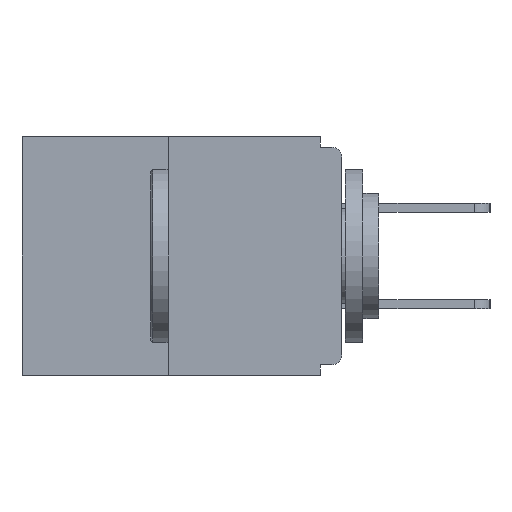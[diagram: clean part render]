
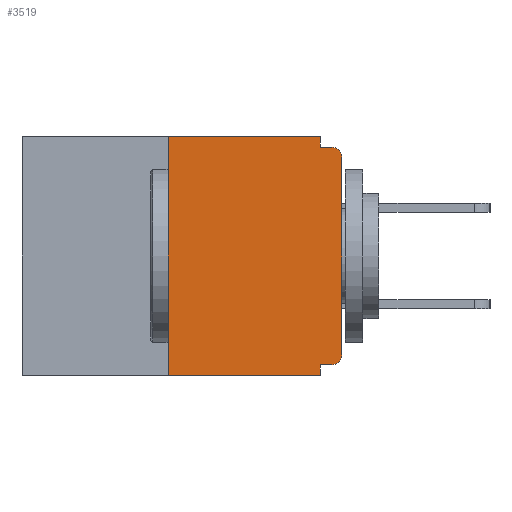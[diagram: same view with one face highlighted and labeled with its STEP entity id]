
A CAD part, left-side view. The second image highlights one B-rep face of the part: STEP entity #3519.
In plain terms, the highlighted planar face has unit normal (-1, 0, 0).
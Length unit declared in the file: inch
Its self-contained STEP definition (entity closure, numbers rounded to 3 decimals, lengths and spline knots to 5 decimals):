
#75 = PLANE ( 'NONE',  #11798 ) ;
#1133 = EDGE_CURVE ( 'NONE', #11866, #6077, #1336, .T. ) ;
#1336 = LINE ( 'NONE', #8271, #6905 ) ;
#1445 = CIRCLE ( 'NONE', #12105, 0.015 ) ;
#1450 = EDGE_CURVE ( 'NONE', #10068, #6450, #13166, .T. ) ;
#1694 = DIRECTION ( 'NONE',  ( 0., 1., 0. ) ) ;
#1868 = AXIS2_PLACEMENT_3D ( 'NONE', #6262, #10805, #14112 ) ;
#1869 = DIRECTION ( 'NONE',  ( -1., 0., 0. ) ) ;
#2560 = CARTESIAN_POINT ( 'NONE',  ( 0., 0., -0.313 ) ) ;
#2639 = ORIENTED_EDGE ( 'NONE', *, *, #13439, .T. ) ;
#2716 = VECTOR ( 'NONE', #14176, 39.37008 ) ;
#2807 = EDGE_LOOP ( 'NONE', ( #3450, #4086, #14605, #4460, #13716, #2639, #9284, #4116, #13426, #13278 ) ) ;
#2814 = CARTESIAN_POINT ( 'NONE',  ( 0., 0.031, 0. ) ) ;
#3253 = VECTOR ( 'NONE', #10194, 39.37008 ) ;
#3293 = LINE ( 'NONE', #13962, #11743 ) ;
#3375 = CARTESIAN_POINT ( 'NONE',  ( 0., 0.25, -0.343 ) ) ;
#3436 = VERTEX_POINT ( 'NONE', #9555 ) ;
#3450 = ORIENTED_EDGE ( 'NONE', *, *, #1450, .F. ) ;
#3519 = ADVANCED_FACE ( 'NONE', ( #8879 ), #75, .F. ) ;
#3564 = DIRECTION ( 'NONE',  ( 0., 0., 1. ) ) ;
#3602 = VERTEX_POINT ( 'NONE', #3375 ) ;
#3792 = CARTESIAN_POINT ( 'NONE',  ( 0., 0.031, -0.343 ) ) ;
#3948 = CARTESIAN_POINT ( 'NONE',  ( 0., 0., -0.015 ) ) ;
#4086 = ORIENTED_EDGE ( 'NONE', *, *, #5072, .F. ) ;
#4116 = ORIENTED_EDGE ( 'NONE', *, *, #10416, .T. ) ;
#4256 = EDGE_CURVE ( 'NONE', #3436, #7676, #9590, .T. ) ;
#4460 = ORIENTED_EDGE ( 'NONE', *, *, #14014, .F. ) ;
#5072 = EDGE_CURVE ( 'NONE', #3602, #10068, #10771, .T. ) ;
#5111 = DIRECTION ( 'NONE',  ( 0., 0., -1. ) ) ;
#5269 = DIRECTION ( 'NONE',  ( 0., 0., -1. ) ) ;
#5365 = VECTOR ( 'NONE', #1694, 39.37008 ) ;
#5390 = VERTEX_POINT ( 'NONE', #5520 ) ;
#5520 = CARTESIAN_POINT ( 'NONE',  ( 0., 0.031, -0.328 ) ) ;
#5783 = DIRECTION ( 'NONE',  ( 1., 0., 0. ) ) ;
#6077 = VERTEX_POINT ( 'NONE', #9287 ) ;
#6115 = EDGE_CURVE ( 'NONE', #11782, #5390, #8964, .T. ) ;
#6226 = DIRECTION ( 'NONE',  ( 0., -1., 0. ) ) ;
#6262 = CARTESIAN_POINT ( 'NONE',  ( 0., 0.015, -0.313 ) ) ;
#6299 = CARTESIAN_POINT ( 'NONE',  ( 0., 0., -0.328 ) ) ;
#6450 = VERTEX_POINT ( 'NONE', #11393 ) ;
#6757 = CARTESIAN_POINT ( 'NONE',  ( 0., 0.46, 0. ) ) ;
#6905 = VECTOR ( 'NONE', #3564, 39.37008 ) ;
#6988 = CARTESIAN_POINT ( 'NONE',  ( 0., 0.46, -0.343 ) ) ;
#7676 = VERTEX_POINT ( 'NONE', #14600 ) ;
#7972 = VECTOR ( 'NONE', #6226, 39.37008 ) ;
#8271 = CARTESIAN_POINT ( 'NONE',  ( 0., 0., 0. ) ) ;
#8824 = CARTESIAN_POINT ( 'NONE',  ( 0., 0.46, 0. ) ) ;
#8879 = FACE_OUTER_BOUND ( 'NONE', #2807, .T. ) ;
#8964 = LINE ( 'NONE', #6299, #5365 ) ;
#9036 = CARTESIAN_POINT ( 'NONE',  ( 0., 0.015, -0.328 ) ) ;
#9061 = EDGE_CURVE ( 'NONE', #3602, #11951, #14658, .T. ) ;
#9284 = ORIENTED_EDGE ( 'NONE', *, *, #1133, .T. ) ;
#9287 = CARTESIAN_POINT ( 'NONE',  ( 0., 0., -0.03 ) ) ;
#9555 = CARTESIAN_POINT ( 'NONE',  ( 0., 0.031, -0.015 ) ) ;
#9590 = LINE ( 'NONE', #3948, #7972 ) ;
#10068 = VERTEX_POINT ( 'NONE', #11251 ) ;
#10194 = DIRECTION ( 'NONE',  ( 0., -1., 0. ) ) ;
#10416 = EDGE_CURVE ( 'NONE', #6077, #7676, #1445, .T. ) ;
#10481 = CIRCLE ( 'NONE', #1868, 0.015 ) ;
#10617 = DIRECTION ( 'NONE',  ( 0., 0., -1. ) ) ;
#10771 = LINE ( 'NONE', #12077, #2716 ) ;
#10805 = DIRECTION ( 'NONE',  ( -1., 0., 0. ) ) ;
#10860 = VECTOR ( 'NONE', #5111, 39.37008 ) ;
#11251 = CARTESIAN_POINT ( 'NONE',  ( 0., 0.25, 0. ) ) ;
#11393 = CARTESIAN_POINT ( 'NONE',  ( 0., 0.031, 0. ) ) ;
#11403 = DIRECTION ( 'NONE',  ( 0., 0., -1. ) ) ;
#11743 = VECTOR ( 'NONE', #10617, 39.37008 ) ;
#11782 = VERTEX_POINT ( 'NONE', #9036 ) ;
#11798 = AXIS2_PLACEMENT_3D ( 'NONE', #6757, #5783, #11403 ) ;
#11866 = VERTEX_POINT ( 'NONE', #2560 ) ;
#11951 = VERTEX_POINT ( 'NONE', #3792 ) ;
#12077 = CARTESIAN_POINT ( 'NONE',  ( 0., 0.25, 0. ) ) ;
#12105 = AXIS2_PLACEMENT_3D ( 'NONE', #12270, #1869, #5269 ) ;
#12270 = CARTESIAN_POINT ( 'NONE',  ( 0., 0.015, -0.03 ) ) ;
#12468 = VECTOR ( 'NONE', #14543, 39.37008 ) ;
#12909 = EDGE_CURVE ( 'NONE', #6450, #3436, #13851, .T. ) ;
#13166 = LINE ( 'NONE', #8824, #12468 ) ;
#13278 = ORIENTED_EDGE ( 'NONE', *, *, #12909, .F. ) ;
#13426 = ORIENTED_EDGE ( 'NONE', *, *, #4256, .F. ) ;
#13439 = EDGE_CURVE ( 'NONE', #11782, #11866, #10481, .T. ) ;
#13716 = ORIENTED_EDGE ( 'NONE', *, *, #6115, .F. ) ;
#13851 = LINE ( 'NONE', #2814, #10860 ) ;
#13962 = CARTESIAN_POINT ( 'NONE',  ( 0., 0.031, -0.343 ) ) ;
#14014 = EDGE_CURVE ( 'NONE', #5390, #11951, #3293, .T. ) ;
#14112 = DIRECTION ( 'NONE',  ( 0., 0., -1. ) ) ;
#14176 = DIRECTION ( 'NONE',  ( 0., 0., 1. ) ) ;
#14543 = DIRECTION ( 'NONE',  ( 0., -1., 0. ) ) ;
#14600 = CARTESIAN_POINT ( 'NONE',  ( 0., 0.015, -0.015 ) ) ;
#14605 = ORIENTED_EDGE ( 'NONE', *, *, #9061, .T. ) ;
#14658 = LINE ( 'NONE', #6988, #3253 ) ;
